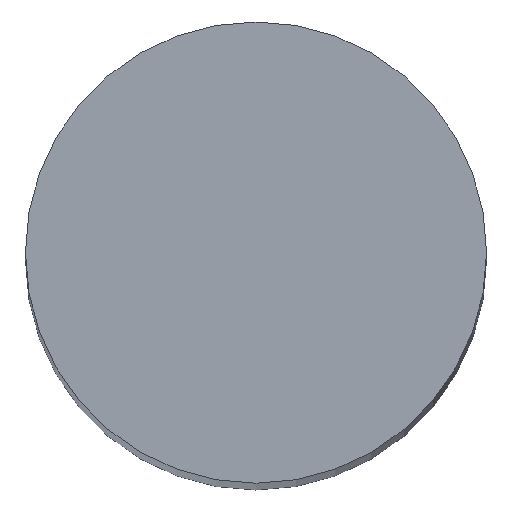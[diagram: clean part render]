
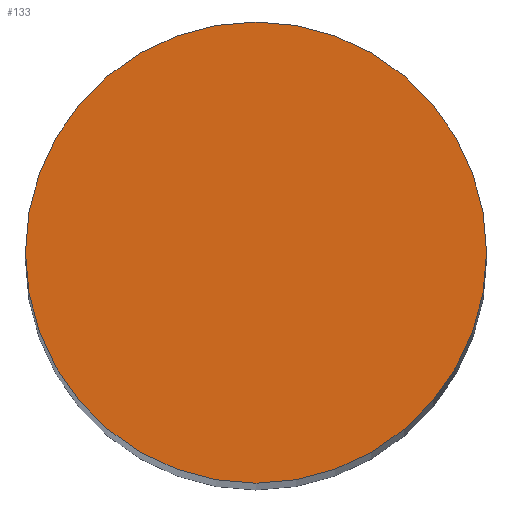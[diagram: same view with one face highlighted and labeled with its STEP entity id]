
A CAD part, top view. The second image highlights one B-rep face of the part: STEP entity #133.
In plain terms, the highlighted planar face has unit normal (0, 0, 1).
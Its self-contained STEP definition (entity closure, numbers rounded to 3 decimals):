
#4 = AXIS2_PLACEMENT_3D ( 'NONE', #80, #60, #10 ) ;
#8 = PLANE ( 'NONE',  #4 ) ;
#10 = DIRECTION ( 'NONE',  ( 1., 0., 0. ) ) ;
#11 = CIRCLE ( 'NONE', #45, 2.413 ) ;
#14 = CARTESIAN_POINT ( 'NONE',  ( 0., 0., 40.64 ) ) ;
#17 = ORIENTED_EDGE ( 'NONE', *, *, #48, .T. ) ;
#20 = DIRECTION ( 'NONE',  ( 1., 0., 0. ) ) ;
#21 = CIRCLE ( 'NONE', #74, 2.413 ) ;
#22 = CARTESIAN_POINT ( 'NONE',  ( -2.413, 0., 40.64 ) ) ;
#28 = ORIENTED_EDGE ( 'NONE', *, *, #78, .T. ) ;
#41 = DIRECTION ( 'NONE',  ( 0., 0., 1. ) ) ;
#43 = VERTEX_POINT ( 'NONE', #51 ) ;
#45 = AXIS2_PLACEMENT_3D ( 'NONE', #122, #41, #105 ) ;
#47 = DIRECTION ( 'NONE',  ( 0., 0., 1. ) ) ;
#48 = EDGE_CURVE ( 'NONE', #43, #77, #11, .T. ) ;
#51 = CARTESIAN_POINT ( 'NONE',  ( 2.413, 0., 40.64 ) ) ;
#60 = DIRECTION ( 'NONE',  ( 0., 0., 1. ) ) ;
#74 = AXIS2_PLACEMENT_3D ( 'NONE', #14, #47, #20 ) ;
#77 = VERTEX_POINT ( 'NONE', #22 ) ;
#78 = EDGE_CURVE ( 'NONE', #77, #43, #21, .T. ) ;
#80 = CARTESIAN_POINT ( 'NONE',  ( 0., 0., 40.64 ) ) ;
#105 = DIRECTION ( 'NONE',  ( 1., 0., 0. ) ) ;
#117 = FACE_OUTER_BOUND ( 'NONE', #120, .T. ) ;
#120 = EDGE_LOOP ( 'NONE', ( #28, #17 ) ) ;
#122 = CARTESIAN_POINT ( 'NONE',  ( 0., 0., 40.64 ) ) ;
#133 = ADVANCED_FACE ( 'NONE', ( #117 ), #8, .T. ) ;
